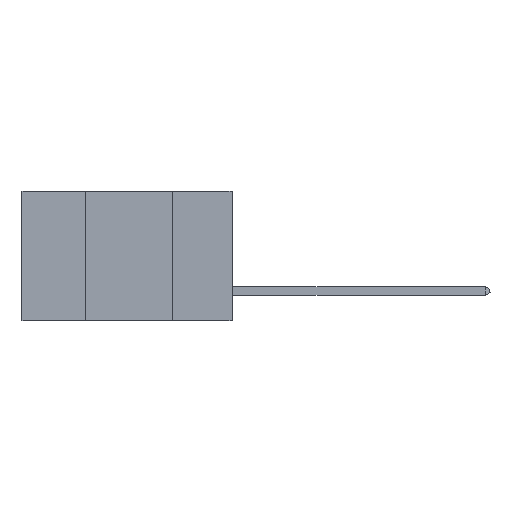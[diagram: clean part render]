
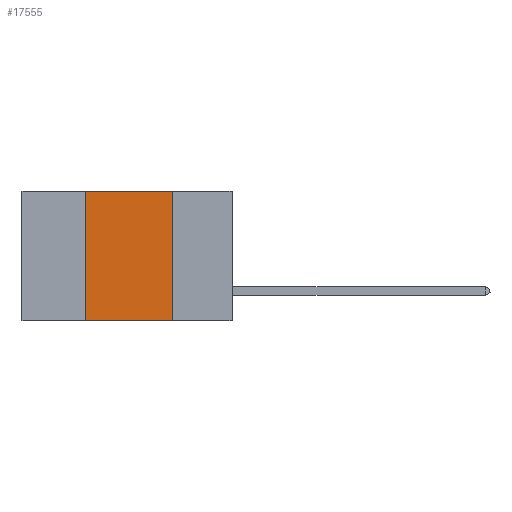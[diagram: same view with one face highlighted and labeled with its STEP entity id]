
A CAD part, left-side view. The second image highlights one B-rep face of the part: STEP entity #17555.
In plain terms, the highlighted planar face has unit normal (-1, 0, 0).
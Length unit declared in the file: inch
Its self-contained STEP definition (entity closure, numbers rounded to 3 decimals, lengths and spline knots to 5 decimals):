
#338 = VERTEX_POINT ( 'NONE', #5693 ) ;
#533 = VECTOR ( 'NONE', #7575, 39.37008 ) ;
#1173 = FACE_OUTER_BOUND ( 'NONE', #25390, .T. ) ;
#1213 = VERTEX_POINT ( 'NONE', #20922 ) ;
#2355 = ORIENTED_EDGE ( 'NONE', *, *, #25457, .T. ) ;
#2736 = PLANE ( 'NONE',  #22781 ) ;
#3445 = DIRECTION ( 'NONE',  ( 0., -1., 0. ) ) ;
#4582 = CARTESIAN_POINT ( 'NONE',  ( 0., 0.17, 0. ) ) ;
#5492 = EDGE_CURVE ( 'NONE', #338, #6294, #23252, .T. ) ;
#5693 = CARTESIAN_POINT ( 'NONE',  ( 0., 0.42, -0.37 ) ) ;
#6294 = VERTEX_POINT ( 'NONE', #8530 ) ;
#6673 = ORIENTED_EDGE ( 'NONE', *, *, #5492, .F. ) ;
#7575 = DIRECTION ( 'NONE',  ( 0., -1., 0. ) ) ;
#8530 = CARTESIAN_POINT ( 'NONE',  ( 0., 0.42, 0. ) ) ;
#8930 = DIRECTION ( 'NONE',  ( 0., 0., -1. ) ) ;
#9489 = ORIENTED_EDGE ( 'NONE', *, *, #23190, .F. ) ;
#10814 = DIRECTION ( 'NONE',  ( 1., 0., 0. ) ) ;
#12253 = EDGE_CURVE ( 'NONE', #14586, #1213, #15388, .T. ) ;
#12276 = LINE ( 'NONE', #17774, #533 ) ;
#14170 = ORIENTED_EDGE ( 'NONE', *, *, #12253, .F. ) ;
#14586 = VERTEX_POINT ( 'NONE', #15424 ) ;
#14653 = CARTESIAN_POINT ( 'NONE',  ( 0., 0.42, 0. ) ) ;
#15388 = LINE ( 'NONE', #4582, #22911 ) ;
#15424 = CARTESIAN_POINT ( 'NONE',  ( 0., 0.17, 0. ) ) ;
#16089 = VECTOR ( 'NONE', #3445, 39.37008 ) ;
#17555 = ADVANCED_FACE ( 'NONE', ( #1173 ), #2736, .F. ) ;
#17774 = CARTESIAN_POINT ( 'NONE',  ( 0., 0.6, 0. ) ) ;
#18662 = DIRECTION ( 'NONE',  ( 0., 0., 1. ) ) ;
#18670 = DIRECTION ( 'NONE',  ( 0., 0., -1. ) ) ;
#20823 = CARTESIAN_POINT ( 'NONE',  ( 0., 0.6, 0. ) ) ;
#20922 = CARTESIAN_POINT ( 'NONE',  ( 0., 0.17, -0.37 ) ) ;
#22033 = LINE ( 'NONE', #23566, #16089 ) ;
#22781 = AXIS2_PLACEMENT_3D ( 'NONE', #20823, #10814, #8930 ) ;
#22897 = VECTOR ( 'NONE', #18662, 39.37008 ) ;
#22911 = VECTOR ( 'NONE', #18670, 39.37008 ) ;
#23190 = EDGE_CURVE ( 'NONE', #6294, #14586, #12276, .T. ) ;
#23252 = LINE ( 'NONE', #14653, #22897 ) ;
#23566 = CARTESIAN_POINT ( 'NONE',  ( 0., 0.6, -0.37 ) ) ;
#25390 = EDGE_LOOP ( 'NONE', ( #14170, #9489, #6673, #2355 ) ) ;
#25457 = EDGE_CURVE ( 'NONE', #338, #1213, #22033, .T. ) ;
